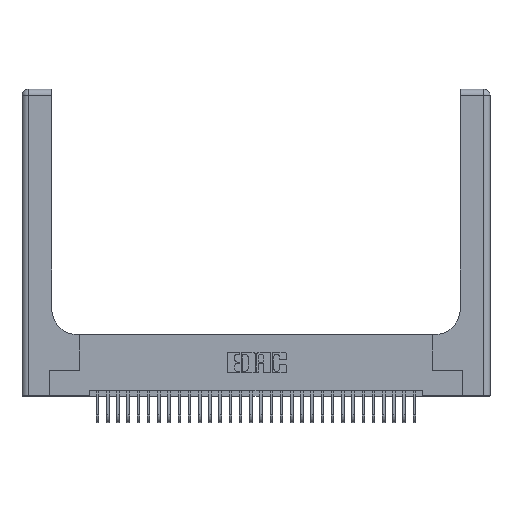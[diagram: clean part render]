
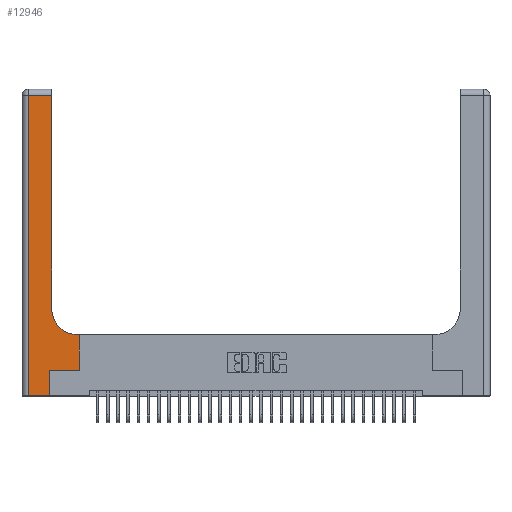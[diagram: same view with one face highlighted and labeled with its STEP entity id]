
A CAD part, top view. The second image highlights one B-rep face of the part: STEP entity #12946.
In plain terms, the highlighted planar face has unit normal (0, 0, 1).
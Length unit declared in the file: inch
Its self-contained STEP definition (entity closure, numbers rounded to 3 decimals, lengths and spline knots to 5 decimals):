
#210 = CARTESIAN_POINT ( 'NONE',  ( 0.269, 0.25, 0.37 ) ) ;
#550 = CARTESIAN_POINT ( 'NONE',  ( 0.269, 0., 0.37 ) ) ;
#1529 = EDGE_CURVE ( 'NONE', #16713, #29721, #6687, .T. ) ;
#1535 = VECTOR ( 'NONE', #18667, 39.37008 ) ;
#1788 = CARTESIAN_POINT ( 'NONE',  ( 0.06, 0., 0.37 ) ) ;
#2107 = CARTESIAN_POINT ( 'NONE',  ( 0., 2.94, 0.37 ) ) ;
#2605 = ORIENTED_EDGE ( 'NONE', *, *, #11232, .T. ) ;
#3645 = CARTESIAN_POINT ( 'NONE',  ( 0.06, 3., 0.37 ) ) ;
#3744 = VERTEX_POINT ( 'NONE', #20931 ) ;
#3856 = CARTESIAN_POINT ( 'NONE',  ( 0.5585, 0.25, 0.37 ) ) ;
#4847 = ORIENTED_EDGE ( 'NONE', *, *, #23621, .T. ) ;
#4923 = VERTEX_POINT ( 'NONE', #19444 ) ;
#5192 = VECTOR ( 'NONE', #28623, 39.37008 ) ;
#5561 = ORIENTED_EDGE ( 'NONE', *, *, #19379, .T. ) ;
#5572 = CARTESIAN_POINT ( 'NONE',  ( 0.2915, 0.6, 0.37 ) ) ;
#5944 = VECTOR ( 'NONE', #15478, 39.37008 ) ;
#6254 = DIRECTION ( 'NONE',  ( 0., 1., 0. ) ) ;
#6387 = FACE_OUTER_BOUND ( 'NONE', #8241, .T. ) ;
#6687 = LINE ( 'NONE', #3645, #5944 ) ;
#7259 = PLANE ( 'NONE',  #18279 ) ;
#7783 = CARTESIAN_POINT ( 'NONE',  ( 0.269, 0., 0.37 ) ) ;
#8241 = EDGE_LOOP ( 'NONE', ( #5561, #24496, #21878, #25636, #2605, #10413, #4847, #26761, #17041 ) ) ;
#8390 = VERTEX_POINT ( 'NONE', #15511 ) ;
#8628 = EDGE_CURVE ( 'NONE', #29721, #10736, #16047, .T. ) ;
#9643 = CARTESIAN_POINT ( 'NONE',  ( 0., 3., 0.37 ) ) ;
#9959 = DIRECTION ( 'NONE',  ( 0., 0., -1. ) ) ;
#10163 = DIRECTION ( 'NONE',  ( 0., 1., 0. ) ) ;
#10413 = ORIENTED_EDGE ( 'NONE', *, *, #13996, .T. ) ;
#10502 = EDGE_CURVE ( 'NONE', #8390, #16713, #26784, .T. ) ;
#10557 = DIRECTION ( 'NONE',  ( 0., 1., 0. ) ) ;
#10581 = LINE ( 'NONE', #7783, #22426 ) ;
#10736 = VERTEX_POINT ( 'NONE', #550 ) ;
#10948 = VERTEX_POINT ( 'NONE', #20535 ) ;
#11232 = EDGE_CURVE ( 'NONE', #10736, #4923, #10581, .T. ) ;
#11522 = LINE ( 'NONE', #210, #5192 ) ;
#11946 = VECTOR ( 'NONE', #10557, 39.37008 ) ;
#12038 = DIRECTION ( 'NONE',  ( -1., 0., 0. ) ) ;
#12946 = ADVANCED_FACE ( 'NONE', ( #6387 ), #7259, .F. ) ;
#13076 = AXIS2_PLACEMENT_3D ( 'NONE', #24163, #9959, #26568 ) ;
#13635 = CARTESIAN_POINT ( 'NONE',  ( 0.06, 2.94, 0.37 ) ) ;
#13810 = CIRCLE ( 'NONE', #13076, 0.25 ) ;
#13996 = EDGE_CURVE ( 'NONE', #4923, #18390, #11522, .T. ) ;
#14499 = LINE ( 'NONE', #3856, #26382 ) ;
#15325 = CARTESIAN_POINT ( 'NONE',  ( 0.2915, 3., 0.37 ) ) ;
#15478 = DIRECTION ( 'NONE',  ( 0., -1., 0. ) ) ;
#15511 = CARTESIAN_POINT ( 'NONE',  ( 0.2915, 2.94, 0.37 ) ) ;
#16047 = LINE ( 'NONE', #25791, #29437 ) ;
#16109 = CARTESIAN_POINT ( 'NONE',  ( 0.5585, 0.6, 0.37 ) ) ;
#16713 = VERTEX_POINT ( 'NONE', #13635 ) ;
#17041 = ORIENTED_EDGE ( 'NONE', *, *, #18608, .T. ) ;
#18279 = AXIS2_PLACEMENT_3D ( 'NONE', #9643, #26245, #12038 ) ;
#18390 = VERTEX_POINT ( 'NONE', #30592 ) ;
#18576 = DIRECTION ( 'NONE',  ( 1., 0., 0. ) ) ;
#18608 = EDGE_CURVE ( 'NONE', #10948, #3744, #13810, .T. ) ;
#18667 = DIRECTION ( 'NONE',  ( -1., 0., 0. ) ) ;
#19379 = EDGE_CURVE ( 'NONE', #3744, #8390, #24560, .T. ) ;
#19444 = CARTESIAN_POINT ( 'NONE',  ( 0.269, 0.25, 0.37 ) ) ;
#19601 = LINE ( 'NONE', #5572, #25181 ) ;
#20535 = CARTESIAN_POINT ( 'NONE',  ( 0.5415, 0.6, 0.37 ) ) ;
#20931 = CARTESIAN_POINT ( 'NONE',  ( 0.2915, 0.85, 0.37 ) ) ;
#21192 = EDGE_CURVE ( 'NONE', #25595, #10948, #19601, .T. ) ;
#21878 = ORIENTED_EDGE ( 'NONE', *, *, #1529, .T. ) ;
#22426 = VECTOR ( 'NONE', #10163, 39.37008 ) ;
#23621 = EDGE_CURVE ( 'NONE', #18390, #25595, #14499, .T. ) ;
#24163 = CARTESIAN_POINT ( 'NONE',  ( 0.5415, 0.85, 0.37 ) ) ;
#24496 = ORIENTED_EDGE ( 'NONE', *, *, #10502, .T. ) ;
#24560 = LINE ( 'NONE', #15325, #11946 ) ;
#25181 = VECTOR ( 'NONE', #29112, 39.37008 ) ;
#25595 = VERTEX_POINT ( 'NONE', #16109 ) ;
#25636 = ORIENTED_EDGE ( 'NONE', *, *, #8628, .T. ) ;
#25791 = CARTESIAN_POINT ( 'NONE',  ( 0., 0., 0.37 ) ) ;
#26245 = DIRECTION ( 'NONE',  ( 0., 0., -1. ) ) ;
#26382 = VECTOR ( 'NONE', #6254, 39.37008 ) ;
#26568 = DIRECTION ( 'NONE',  ( 1., 0., 0. ) ) ;
#26761 = ORIENTED_EDGE ( 'NONE', *, *, #21192, .T. ) ;
#26784 = LINE ( 'NONE', #2107, #1535 ) ;
#28623 = DIRECTION ( 'NONE',  ( 1., 0., 0. ) ) ;
#29112 = DIRECTION ( 'NONE',  ( -1., 0., 0. ) ) ;
#29437 = VECTOR ( 'NONE', #18576, 39.37008 ) ;
#29721 = VERTEX_POINT ( 'NONE', #1788 ) ;
#30592 = CARTESIAN_POINT ( 'NONE',  ( 0.5585, 0.25, 0.37 ) ) ;
